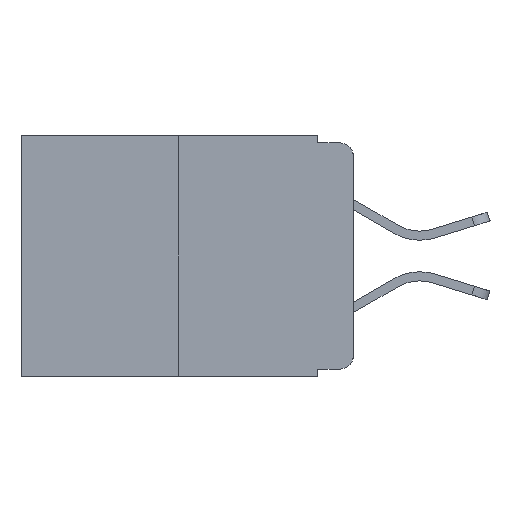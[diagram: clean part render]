
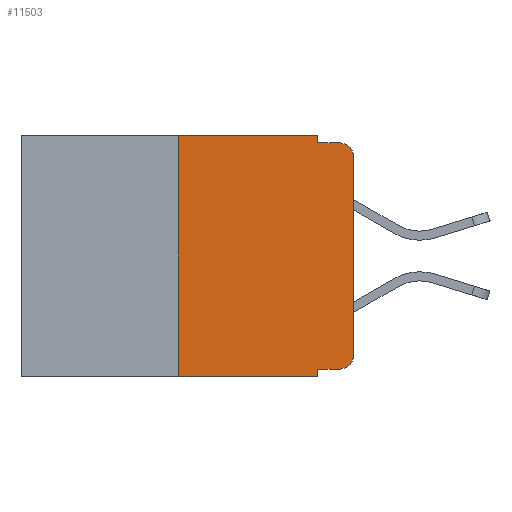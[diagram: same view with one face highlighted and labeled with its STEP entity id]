
A CAD part, left-side view. The second image highlights one B-rep face of the part: STEP entity #11503.
In plain terms, the highlighted planar face has unit normal (-1, 0, 0).
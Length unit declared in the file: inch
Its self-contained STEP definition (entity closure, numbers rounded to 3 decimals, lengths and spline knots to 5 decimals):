
#45 = ORIENTED_EDGE ( 'NONE', *, *, #16713, .T. ) ;
#271 = EDGE_CURVE ( 'NONE', #2297, #7325, #6072, .T. ) ;
#625 = CARTESIAN_POINT ( 'NONE',  ( 0., 0.02, -0.01 ) ) ;
#715 = LINE ( 'NONE', #9346, #13149 ) ;
#840 = DIRECTION ( 'NONE',  ( 0., -1., 0. ) ) ;
#944 = CARTESIAN_POINT ( 'NONE',  ( 0., 0.25, 0. ) ) ;
#970 = CARTESIAN_POINT ( 'NONE',  ( 0., 0.473, -0.343 ) ) ;
#985 = CARTESIAN_POINT ( 'NONE',  ( 0., 0.02, -0.333 ) ) ;
#1028 = ORIENTED_EDGE ( 'NONE', *, *, #16749, .T. ) ;
#1233 = VECTOR ( 'NONE', #4625, 39.37008 ) ;
#1658 = FACE_OUTER_BOUND ( 'NONE', #8768, .T. ) ;
#1684 = CIRCLE ( 'NONE', #4872, 0.02 ) ;
#2134 = VERTEX_POINT ( 'NONE', #625 ) ;
#2297 = VERTEX_POINT ( 'NONE', #10305 ) ;
#2351 = ORIENTED_EDGE ( 'NONE', *, *, #2440, .F. ) ;
#2440 = EDGE_CURVE ( 'NONE', #5791, #15328, #715, .T. ) ;
#2478 = CARTESIAN_POINT ( 'NONE',  ( 0., 0.051, 0. ) ) ;
#2497 = DIRECTION ( 'NONE',  ( 0., 0., 1. ) ) ;
#3436 = DIRECTION ( 'NONE',  ( -1., 0., 0. ) ) ;
#3898 = ORIENTED_EDGE ( 'NONE', *, *, #16862, .F. ) ;
#4288 = VECTOR ( 'NONE', #7079, 39.37008 ) ;
#4494 = CARTESIAN_POINT ( 'NONE',  ( 0., 0.051, -0.343 ) ) ;
#4625 = DIRECTION ( 'NONE',  ( 0., 0., 1. ) ) ;
#4644 = CARTESIAN_POINT ( 'NONE',  ( 0., 0.051, 0. ) ) ;
#4872 = AXIS2_PLACEMENT_3D ( 'NONE', #12574, #3436, #17213 ) ;
#5078 = EDGE_CURVE ( 'NONE', #12840, #2134, #6133, .T. ) ;
#5120 = CARTESIAN_POINT ( 'NONE',  ( 0., 0.051, -0.333 ) ) ;
#5741 = CARTESIAN_POINT ( 'NONE',  ( 0., 0., -0.03 ) ) ;
#5791 = VERTEX_POINT ( 'NONE', #19839 ) ;
#6072 = LINE ( 'NONE', #14143, #16330 ) ;
#6133 = LINE ( 'NONE', #8583, #10647 ) ;
#6346 = VERTEX_POINT ( 'NONE', #5741 ) ;
#6486 = DIRECTION ( 'NONE',  ( 0., -1., 0. ) ) ;
#6849 = EDGE_CURVE ( 'NONE', #6346, #2134, #14027, .T. ) ;
#7079 = DIRECTION ( 'NONE',  ( 0., 0., -1. ) ) ;
#7241 = ORIENTED_EDGE ( 'NONE', *, *, #17564, .F. ) ;
#7325 = VERTEX_POINT ( 'NONE', #4644 ) ;
#8452 = AXIS2_PLACEMENT_3D ( 'NONE', #14637, #9904, #8559 ) ;
#8559 = DIRECTION ( 'NONE',  ( 0., 0., -1. ) ) ;
#8583 = CARTESIAN_POINT ( 'NONE',  ( 0., 0.051, -0.01 ) ) ;
#8768 = EDGE_LOOP ( 'NONE', ( #19677, #13032, #15665, #7241, #15942, #3898, #9691, #2351, #45, #1028 ) ) ;
#9073 = EDGE_CURVE ( 'NONE', #17891, #15328, #13451, .T. ) ;
#9346 = CARTESIAN_POINT ( 'NONE',  ( 0., 0.051, 0. ) ) ;
#9691 = ORIENTED_EDGE ( 'NONE', *, *, #9073, .T. ) ;
#9720 = CARTESIAN_POINT ( 'NONE',  ( 0., 0.25, -0.343 ) ) ;
#9777 = VECTOR ( 'NONE', #2497, 39.37008 ) ;
#9904 = DIRECTION ( 'NONE',  ( 1., 0., 0. ) ) ;
#10305 = CARTESIAN_POINT ( 'NONE',  ( 0., 0.25, 0. ) ) ;
#10359 = CARTESIAN_POINT ( 'NONE',  ( 0., 0., -0.313 ) ) ;
#10462 = CARTESIAN_POINT ( 'NONE',  ( 0., 0.051, -0.01 ) ) ;
#10618 = CARTESIAN_POINT ( 'NONE',  ( 0., 0., 0. ) ) ;
#10647 = VECTOR ( 'NONE', #840, 39.37008 ) ;
#11231 = LINE ( 'NONE', #944, #9777 ) ;
#11384 = DIRECTION ( 'NONE',  ( 0., -1., 0. ) ) ;
#11503 = ADVANCED_FACE ( 'NONE', ( #1658 ), #11633, .F. ) ;
#11633 = PLANE ( 'NONE',  #8452 ) ;
#11679 = VERTEX_POINT ( 'NONE', #10359 ) ;
#12012 = AXIS2_PLACEMENT_3D ( 'NONE', #13101, #16580, #16350 ) ;
#12574 = CARTESIAN_POINT ( 'NONE',  ( 0., 0.02, -0.313 ) ) ;
#12840 = VERTEX_POINT ( 'NONE', #10462 ) ;
#12885 = VECTOR ( 'NONE', #15777, 39.37008 ) ;
#13032 = ORIENTED_EDGE ( 'NONE', *, *, #6849, .T. ) ;
#13101 = CARTESIAN_POINT ( 'NONE',  ( 0., 0.02, -0.03 ) ) ;
#13149 = VECTOR ( 'NONE', #13948, 39.37008 ) ;
#13451 = LINE ( 'NONE', #970, #17807 ) ;
#13948 = DIRECTION ( 'NONE',  ( 0., 0., -1. ) ) ;
#14027 = CIRCLE ( 'NONE', #12012, 0.02 ) ;
#14064 = LINE ( 'NONE', #2478, #4288 ) ;
#14143 = CARTESIAN_POINT ( 'NONE',  ( 0., 0.473, 0. ) ) ;
#14637 = CARTESIAN_POINT ( 'NONE',  ( 0., 0.473, 0. ) ) ;
#15270 = EDGE_CURVE ( 'NONE', #11679, #6346, #18475, .T. ) ;
#15328 = VERTEX_POINT ( 'NONE', #4494 ) ;
#15665 = ORIENTED_EDGE ( 'NONE', *, *, #5078, .F. ) ;
#15771 = LINE ( 'NONE', #5120, #12885 ) ;
#15777 = DIRECTION ( 'NONE',  ( 0., -1., 0. ) ) ;
#15942 = ORIENTED_EDGE ( 'NONE', *, *, #271, .F. ) ;
#16330 = VECTOR ( 'NONE', #6486, 39.37008 ) ;
#16350 = DIRECTION ( 'NONE',  ( 0., 0., -1. ) ) ;
#16580 = DIRECTION ( 'NONE',  ( -1., 0., 0. ) ) ;
#16713 = EDGE_CURVE ( 'NONE', #5791, #19432, #15771, .T. ) ;
#16749 = EDGE_CURVE ( 'NONE', #19432, #11679, #1684, .T. ) ;
#16862 = EDGE_CURVE ( 'NONE', #17891, #2297, #11231, .T. ) ;
#17213 = DIRECTION ( 'NONE',  ( 0., 0., -1. ) ) ;
#17564 = EDGE_CURVE ( 'NONE', #7325, #12840, #14064, .T. ) ;
#17807 = VECTOR ( 'NONE', #11384, 39.37008 ) ;
#17891 = VERTEX_POINT ( 'NONE', #9720 ) ;
#18475 = LINE ( 'NONE', #10618, #1233 ) ;
#19432 = VERTEX_POINT ( 'NONE', #985 ) ;
#19677 = ORIENTED_EDGE ( 'NONE', *, *, #15270, .T. ) ;
#19839 = CARTESIAN_POINT ( 'NONE',  ( 0., 0.051, -0.333 ) ) ;
